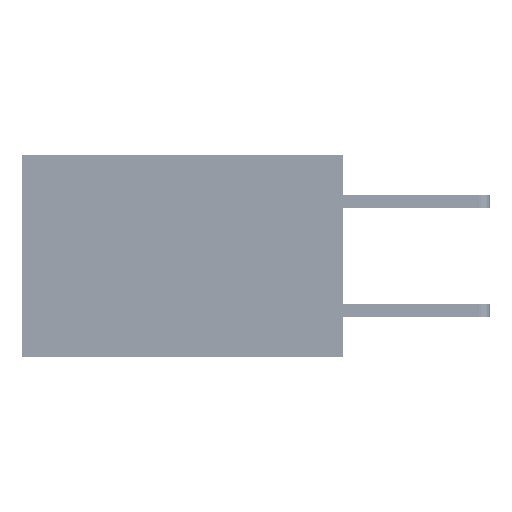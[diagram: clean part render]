
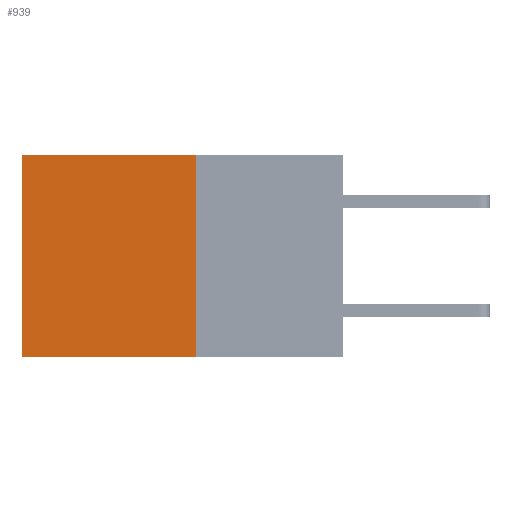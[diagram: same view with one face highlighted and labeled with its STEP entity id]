
A CAD part, left-side view. The second image highlights one B-rep face of the part: STEP entity #939.
In plain terms, the highlighted planar face has unit normal (-1, 0, 0).
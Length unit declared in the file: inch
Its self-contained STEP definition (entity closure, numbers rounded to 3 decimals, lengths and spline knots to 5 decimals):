
#12 = DIRECTION ( 'NONE',  ( 1., 0., 0. ) ) ;
#939 = ADVANCED_FACE ( 'NONE', ( #25265 ), #4840, .F. ) ;
#1579 = LINE ( 'NONE', #15811, #16422 ) ;
#2392 = EDGE_CURVE ( 'NONE', #29995, #6322, #7949, .T. ) ;
#4840 = PLANE ( 'NONE',  #14318 ) ;
#6322 = VERTEX_POINT ( 'NONE', #27928 ) ;
#7949 = LINE ( 'NONE', #18141, #21775 ) ;
#8853 = DIRECTION ( 'NONE',  ( 0., 0., -1. ) ) ;
#9323 = VECTOR ( 'NONE', #8853, 39.37008 ) ;
#10458 = CARTESIAN_POINT ( 'NONE',  ( 0.277, 0.59, -0.37 ) ) ;
#11408 = CARTESIAN_POINT ( 'NONE',  ( 0.277, 0.27, -0.37 ) ) ;
#12614 = ORIENTED_EDGE ( 'NONE', *, *, #2392, .F. ) ;
#14318 = AXIS2_PLACEMENT_3D ( 'NONE', #29726, #12, #33205 ) ;
#15811 = CARTESIAN_POINT ( 'NONE',  ( 0.277, 0.27, 0. ) ) ;
#16422 = VECTOR ( 'NONE', #18534, 39.37008 ) ;
#16955 = DIRECTION ( 'NONE',  ( 0., 1., 0. ) ) ;
#17085 = ORIENTED_EDGE ( 'NONE', *, *, #26989, .T. ) ;
#17948 = VERTEX_POINT ( 'NONE', #26174 ) ;
#18141 = CARTESIAN_POINT ( 'NONE',  ( 0.277, 0.27, -0.37 ) ) ;
#18534 = DIRECTION ( 'NONE',  ( 0., 1., 0. ) ) ;
#19685 = EDGE_CURVE ( 'NONE', #6322, #23012, #27915, .T. ) ;
#19853 = CARTESIAN_POINT ( 'NONE',  ( 0.277, 0.59, -0.37 ) ) ;
#21775 = VECTOR ( 'NONE', #34543, 39.37008 ) ;
#22005 = ORIENTED_EDGE ( 'NONE', *, *, #19685, .F. ) ;
#23012 = VERTEX_POINT ( 'NONE', #10458 ) ;
#23943 = LINE ( 'NONE', #19853, #9323 ) ;
#25265 = FACE_OUTER_BOUND ( 'NONE', #33066, .T. ) ;
#26174 = CARTESIAN_POINT ( 'NONE',  ( 0.277, 0.59, 0. ) ) ;
#26989 = EDGE_CURVE ( 'NONE', #29995, #17948, #1579, .T. ) ;
#27481 = ORIENTED_EDGE ( 'NONE', *, *, #28962, .T. ) ;
#27915 = LINE ( 'NONE', #11408, #35240 ) ;
#27928 = CARTESIAN_POINT ( 'NONE',  ( 0.277, 0.27, -0.37 ) ) ;
#28962 = EDGE_CURVE ( 'NONE', #17948, #23012, #23943, .T. ) ;
#29186 = CARTESIAN_POINT ( 'NONE',  ( 0.277, 0.27, 0. ) ) ;
#29726 = CARTESIAN_POINT ( 'NONE',  ( 0.277, 0.27, -0.37 ) ) ;
#29995 = VERTEX_POINT ( 'NONE', #29186 ) ;
#33066 = EDGE_LOOP ( 'NONE', ( #27481, #22005, #12614, #17085 ) ) ;
#33205 = DIRECTION ( 'NONE',  ( 0., 0., -1. ) ) ;
#34543 = DIRECTION ( 'NONE',  ( 0., 0., -1. ) ) ;
#35240 = VECTOR ( 'NONE', #16955, 39.37008 ) ;
